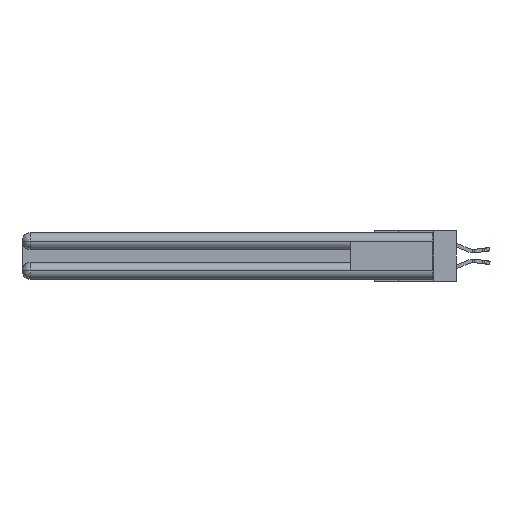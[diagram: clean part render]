
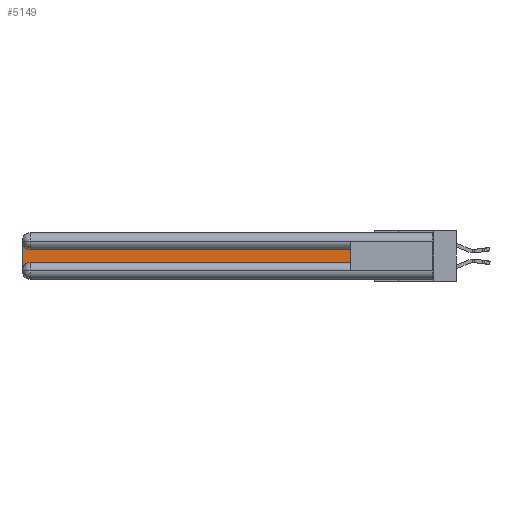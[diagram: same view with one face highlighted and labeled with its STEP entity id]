
A CAD part, left-side view. The second image highlights one B-rep face of the part: STEP entity #5149.
In plain terms, the highlighted planar face has unit normal (-1, 0, 0).
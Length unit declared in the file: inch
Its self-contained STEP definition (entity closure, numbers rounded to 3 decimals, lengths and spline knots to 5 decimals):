
#404 = VERTEX_POINT ( 'NONE', #6840 ) ;
#425 = VECTOR ( 'NONE', #13173, 39.37008 ) ;
#779 = EDGE_CURVE ( 'NONE', #20672, #32585, #14603, .T. ) ;
#1015 = DIRECTION ( 'NONE',  ( 1., 0., 0. ) ) ;
#1241 = EDGE_LOOP ( 'NONE', ( #11903, #10087, #15181, #26029, #20885, #30057 ) ) ;
#1395 = AXIS2_PLACEMENT_3D ( 'NONE', #19808, #27289, #4506 ) ;
#2621 = CARTESIAN_POINT ( 'NONE',  ( 0.075, 3., -0.2175 ) ) ;
#3646 = CARTESIAN_POINT ( 'NONE',  ( 0.075, 0.6, -0.2175 ) ) ;
#3793 = CARTESIAN_POINT ( 'NONE',  ( 0.075, 2.94, -0.1225 ) ) ;
#4506 = DIRECTION ( 'NONE',  ( 0., 0., -1. ) ) ;
#5072 = DIRECTION ( 'NONE',  ( 0., 0., -1. ) ) ;
#5149 = ADVANCED_FACE ( 'NONE', ( #32297 ), #32990, .F. ) ;
#5353 = EDGE_CURVE ( 'NONE', #30569, #20672, #19840, .T. ) ;
#6840 = CARTESIAN_POINT ( 'NONE',  ( 0.075, 3., -0.0625 ) ) ;
#9969 = EDGE_CURVE ( 'NONE', #404, #21695, #13959, .T. ) ;
#10087 = ORIENTED_EDGE ( 'NONE', *, *, #27584, .T. ) ;
#10873 = CIRCLE ( 'NONE', #1395, 0.06 ) ;
#11887 = VECTOR ( 'NONE', #23337, 39.37008 ) ;
#11903 = ORIENTED_EDGE ( 'NONE', *, *, #779, .T. ) ;
#12794 = CARTESIAN_POINT ( 'NONE',  ( 0.075, 3., -0.1225 ) ) ;
#13173 = DIRECTION ( 'NONE',  ( 0., -1., 0. ) ) ;
#13413 = VECTOR ( 'NONE', #17667, 39.37008 ) ;
#13959 = LINE ( 'NONE', #2621, #31967 ) ;
#14603 = LINE ( 'NONE', #29649, #13413 ) ;
#15181 = ORIENTED_EDGE ( 'NONE', *, *, #9969, .T. ) ;
#15864 = VERTEX_POINT ( 'NONE', #20890 ) ;
#17667 = DIRECTION ( 'NONE',  ( 0., 1., 0. ) ) ;
#17916 = AXIS2_PLACEMENT_3D ( 'NONE', #12794, #30663, #28270 ) ;
#18169 = CARTESIAN_POINT ( 'NONE',  ( 0.075, 0.6, -0.2175 ) ) ;
#18507 = CARTESIAN_POINT ( 'NONE',  ( 0.075, 0.6, -0.1225 ) ) ;
#19808 = CARTESIAN_POINT ( 'NONE',  ( 0.075, 2.94, -0.0625 ) ) ;
#19840 = LINE ( 'NONE', #22349, #11887 ) ;
#20672 = VERTEX_POINT ( 'NONE', #18507 ) ;
#20885 = ORIENTED_EDGE ( 'NONE', *, *, #28981, .T. ) ;
#20890 = CARTESIAN_POINT ( 'NONE',  ( 0.075, 2.94, -0.2175 ) ) ;
#21378 = CARTESIAN_POINT ( 'NONE',  ( 0.075, 2.94, -0.2775 ) ) ;
#21477 = DIRECTION ( 'NONE',  ( 0., 0., -1. ) ) ;
#21695 = VERTEX_POINT ( 'NONE', #32960 ) ;
#22349 = CARTESIAN_POINT ( 'NONE',  ( 0.075, 0.6, -0.2175 ) ) ;
#23191 = EDGE_CURVE ( 'NONE', #21695, #15864, #23219, .T. ) ;
#23206 = LINE ( 'NONE', #18169, #425 ) ;
#23219 = CIRCLE ( 'NONE', #30462, 0.06 ) ;
#23337 = DIRECTION ( 'NONE',  ( 0., 0., 1. ) ) ;
#26029 = ORIENTED_EDGE ( 'NONE', *, *, #23191, .T. ) ;
#27289 = DIRECTION ( 'NONE',  ( 1., 0., 0. ) ) ;
#27584 = EDGE_CURVE ( 'NONE', #32585, #404, #10873, .T. ) ;
#28270 = DIRECTION ( 'NONE',  ( 0., 0., -1. ) ) ;
#28981 = EDGE_CURVE ( 'NONE', #15864, #30569, #23206, .T. ) ;
#29649 = CARTESIAN_POINT ( 'NONE',  ( 0.075, 0.6, -0.1225 ) ) ;
#30057 = ORIENTED_EDGE ( 'NONE', *, *, #5353, .T. ) ;
#30462 = AXIS2_PLACEMENT_3D ( 'NONE', #21378, #1015, #21477 ) ;
#30569 = VERTEX_POINT ( 'NONE', #3646 ) ;
#30663 = DIRECTION ( 'NONE',  ( 1., 0., 0. ) ) ;
#31967 = VECTOR ( 'NONE', #5072, 39.37008 ) ;
#32297 = FACE_OUTER_BOUND ( 'NONE', #1241, .T. ) ;
#32585 = VERTEX_POINT ( 'NONE', #3793 ) ;
#32960 = CARTESIAN_POINT ( 'NONE',  ( 0.075, 3., -0.2775 ) ) ;
#32990 = PLANE ( 'NONE',  #17916 ) ;
